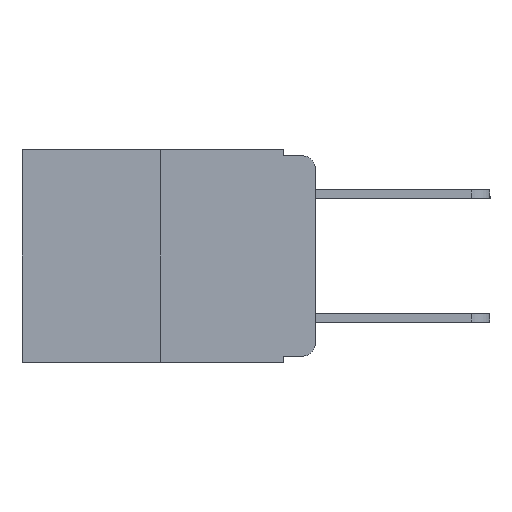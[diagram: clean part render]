
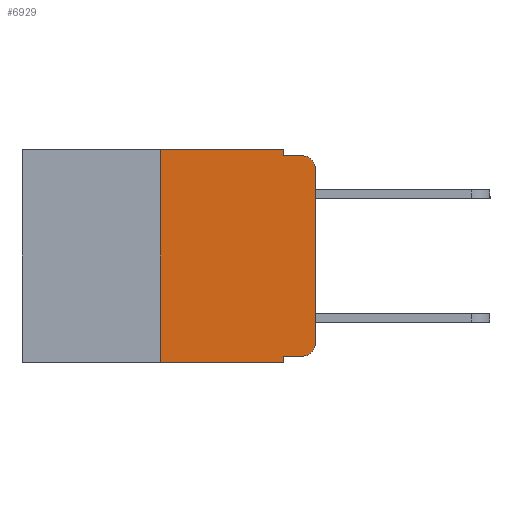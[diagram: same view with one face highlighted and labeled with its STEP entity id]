
A CAD part, left-side view. The second image highlights one B-rep face of the part: STEP entity #6929.
In plain terms, the highlighted planar face has unit normal (-1, 0, 0).
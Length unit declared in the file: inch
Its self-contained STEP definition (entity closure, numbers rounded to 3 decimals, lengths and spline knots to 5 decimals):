
#12 = EDGE_CURVE ( 'NONE', #8489, #4135, #10032, .T. ) ;
#358 = EDGE_CURVE ( 'NONE', #9973, #428, #3124, .T. ) ;
#377 = LINE ( 'NONE', #2647, #713 ) ;
#428 = VERTEX_POINT ( 'NONE', #4075 ) ;
#468 = EDGE_CURVE ( 'NONE', #9973, #9562, #1708, .T. ) ;
#530 = CARTESIAN_POINT ( 'NONE',  ( 0., 0., -0.313 ) ) ;
#713 = VECTOR ( 'NONE', #6945, 39.37008 ) ;
#802 = CARTESIAN_POINT ( 'NONE',  ( 0., 0.051, 0. ) ) ;
#1041 = LINE ( 'NONE', #4097, #7963 ) ;
#1110 = VECTOR ( 'NONE', #8798, 39.37008 ) ;
#1309 = VERTEX_POINT ( 'NONE', #8429 ) ;
#1708 = LINE ( 'NONE', #8095, #1110 ) ;
#1860 = EDGE_CURVE ( 'NONE', #4135, #6133, #5392, .T. ) ;
#1877 = VERTEX_POINT ( 'NONE', #6378 ) ;
#1890 = FACE_OUTER_BOUND ( 'NONE', #5481, .T. ) ;
#2256 = DIRECTION ( 'NONE',  ( -1., 0., 0. ) ) ;
#2466 = AXIS2_PLACEMENT_3D ( 'NONE', #4814, #2256, #2484 ) ;
#2484 = DIRECTION ( 'NONE',  ( 0., 0., -1. ) ) ;
#2647 = CARTESIAN_POINT ( 'NONE',  ( 0., 0.051, -0.01 ) ) ;
#2842 = DIRECTION ( 'NONE',  ( 0., 0., -1. ) ) ;
#2980 = VECTOR ( 'NONE', #8604, 39.37008 ) ;
#3124 = LINE ( 'NONE', #802, #7148 ) ;
#3607 = AXIS2_PLACEMENT_3D ( 'NONE', #7229, #7179, #10763 ) ;
#3842 = CARTESIAN_POINT ( 'NONE',  ( 0., 0.051, 0. ) ) ;
#4059 = PLANE ( 'NONE',  #8886 ) ;
#4075 = CARTESIAN_POINT ( 'NONE',  ( 0., 0.051, -0.343 ) ) ;
#4097 = CARTESIAN_POINT ( 'NONE',  ( 0., 0.051, 0. ) ) ;
#4135 = VERTEX_POINT ( 'NONE', #9995 ) ;
#4308 = EDGE_CURVE ( 'NONE', #9562, #10598, #5349, .T. ) ;
#4534 = DIRECTION ( 'NONE',  ( 0., 0., -1. ) ) ;
#4814 = CARTESIAN_POINT ( 'NONE',  ( 0., 0.02, -0.03 ) ) ;
#4828 = VERTEX_POINT ( 'NONE', #4875 ) ;
#4875 = CARTESIAN_POINT ( 'NONE',  ( 0., 0., -0.03 ) ) ;
#5040 = EDGE_CURVE ( 'NONE', #8489, #428, #5729, .T. ) ;
#5086 = ORIENTED_EDGE ( 'NONE', *, *, #5168, .F. ) ;
#5168 = EDGE_CURVE ( 'NONE', #6133, #1309, #1041, .T. ) ;
#5216 = CARTESIAN_POINT ( 'NONE',  ( 0., 0., 0. ) ) ;
#5349 = CIRCLE ( 'NONE', #3607, 0.02 ) ;
#5392 = LINE ( 'NONE', #10485, #2980 ) ;
#5481 = EDGE_LOOP ( 'NONE', ( #7072, #7239, #8746, #5086, #8529, #10568, #10604, #10266, #10161, #9313 ) ) ;
#5607 = CIRCLE ( 'NONE', #2466, 0.02 ) ;
#5729 = LINE ( 'NONE', #6734, #9627 ) ;
#5880 = EDGE_CURVE ( 'NONE', #10598, #4828, #9829, .T. ) ;
#6133 = VERTEX_POINT ( 'NONE', #3842 ) ;
#6178 = VECTOR ( 'NONE', #9050, 39.37008 ) ;
#6378 = CARTESIAN_POINT ( 'NONE',  ( 0., 0.02, -0.01 ) ) ;
#6734 = CARTESIAN_POINT ( 'NONE',  ( 0., 0.473, -0.343 ) ) ;
#6929 = ADVANCED_FACE ( 'NONE', ( #1890 ), #4059, .F. ) ;
#6945 = DIRECTION ( 'NONE',  ( 0., -1., 0. ) ) ;
#7072 = ORIENTED_EDGE ( 'NONE', *, *, #5880, .T. ) ;
#7083 = DIRECTION ( 'NONE',  ( 0., 0., 1. ) ) ;
#7148 = VECTOR ( 'NONE', #9384, 39.37008 ) ;
#7179 = DIRECTION ( 'NONE',  ( -1., 0., 0. ) ) ;
#7229 = CARTESIAN_POINT ( 'NONE',  ( 0., 0.02, -0.313 ) ) ;
#7239 = ORIENTED_EDGE ( 'NONE', *, *, #8150, .T. ) ;
#7555 = VECTOR ( 'NONE', #7083, 39.37008 ) ;
#7562 = CARTESIAN_POINT ( 'NONE',  ( 0., 0.473, 0. ) ) ;
#7852 = CARTESIAN_POINT ( 'NONE',  ( 0., 0.25, 0. ) ) ;
#7928 = DIRECTION ( 'NONE',  ( 1., 0., 0. ) ) ;
#7963 = VECTOR ( 'NONE', #4534, 39.37008 ) ;
#8095 = CARTESIAN_POINT ( 'NONE',  ( 0., 0.051, -0.333 ) ) ;
#8139 = CARTESIAN_POINT ( 'NONE',  ( 0., 0.25, -0.343 ) ) ;
#8150 = EDGE_CURVE ( 'NONE', #4828, #1877, #5607, .T. ) ;
#8160 = EDGE_CURVE ( 'NONE', #1309, #1877, #377, .T. ) ;
#8429 = CARTESIAN_POINT ( 'NONE',  ( 0., 0.051, -0.01 ) ) ;
#8489 = VERTEX_POINT ( 'NONE', #8139 ) ;
#8529 = ORIENTED_EDGE ( 'NONE', *, *, #1860, .F. ) ;
#8604 = DIRECTION ( 'NONE',  ( 0., -1., 0. ) ) ;
#8746 = ORIENTED_EDGE ( 'NONE', *, *, #8160, .F. ) ;
#8798 = DIRECTION ( 'NONE',  ( 0., -1., 0. ) ) ;
#8886 = AXIS2_PLACEMENT_3D ( 'NONE', #7562, #7928, #2842 ) ;
#8901 = CARTESIAN_POINT ( 'NONE',  ( 0., 0.02, -0.333 ) ) ;
#9050 = DIRECTION ( 'NONE',  ( 0., 0., 1. ) ) ;
#9124 = DIRECTION ( 'NONE',  ( 0., -1., 0. ) ) ;
#9313 = ORIENTED_EDGE ( 'NONE', *, *, #4308, .T. ) ;
#9384 = DIRECTION ( 'NONE',  ( 0., 0., -1. ) ) ;
#9562 = VERTEX_POINT ( 'NONE', #8901 ) ;
#9627 = VECTOR ( 'NONE', #9124, 39.37008 ) ;
#9829 = LINE ( 'NONE', #5216, #7555 ) ;
#9973 = VERTEX_POINT ( 'NONE', #10958 ) ;
#9995 = CARTESIAN_POINT ( 'NONE',  ( 0., 0.25, 0. ) ) ;
#10032 = LINE ( 'NONE', #7852, #6178 ) ;
#10161 = ORIENTED_EDGE ( 'NONE', *, *, #468, .T. ) ;
#10266 = ORIENTED_EDGE ( 'NONE', *, *, #358, .F. ) ;
#10485 = CARTESIAN_POINT ( 'NONE',  ( 0., 0.473, 0. ) ) ;
#10568 = ORIENTED_EDGE ( 'NONE', *, *, #12, .F. ) ;
#10598 = VERTEX_POINT ( 'NONE', #530 ) ;
#10604 = ORIENTED_EDGE ( 'NONE', *, *, #5040, .T. ) ;
#10763 = DIRECTION ( 'NONE',  ( 0., 0., -1. ) ) ;
#10958 = CARTESIAN_POINT ( 'NONE',  ( 0., 0.051, -0.333 ) ) ;
